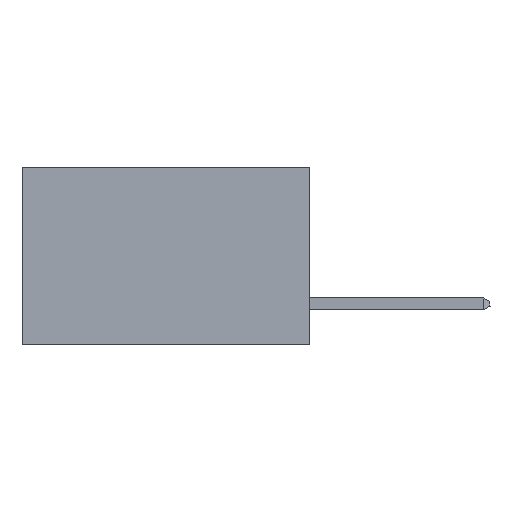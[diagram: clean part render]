
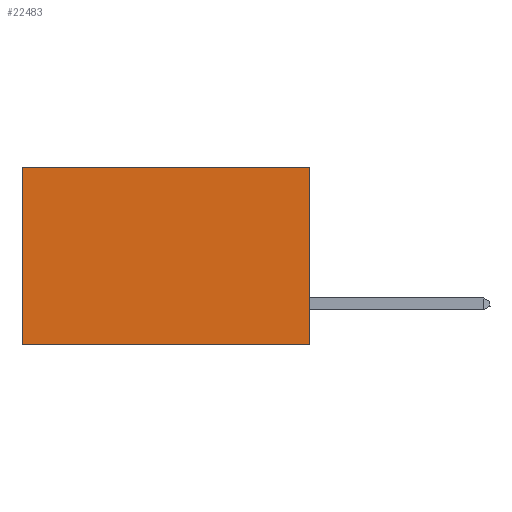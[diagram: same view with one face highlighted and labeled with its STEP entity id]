
A CAD part, left-side view. The second image highlights one B-rep face of the part: STEP entity #22483.
In plain terms, the highlighted planar face has unit normal (-1, 0, 0).
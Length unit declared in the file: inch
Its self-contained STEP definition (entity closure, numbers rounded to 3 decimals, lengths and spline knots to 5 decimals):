
#143 = EDGE_CURVE ( 'NONE', #15144, #19275, #2142, .T. ) ;
#1779 = CARTESIAN_POINT ( 'NONE',  ( 0.2875, 0., 0. ) ) ;
#2142 = LINE ( 'NONE', #35405, #35036 ) ;
#3625 = CARTESIAN_POINT ( 'NONE',  ( 0.2875, 0., 0. ) ) ;
#3890 = CARTESIAN_POINT ( 'NONE',  ( 0.2875, 0.6, 0. ) ) ;
#4076 = VECTOR ( 'NONE', #26128, 39.37008 ) ;
#5432 = ORIENTED_EDGE ( 'NONE', *, *, #30494, .T. ) ;
#9721 = LINE ( 'NONE', #30289, #23962 ) ;
#9836 = ORIENTED_EDGE ( 'NONE', *, *, #143, .F. ) ;
#10707 = DIRECTION ( 'NONE',  ( 0., 0., -1. ) ) ;
#11619 = LINE ( 'NONE', #17474, #4076 ) ;
#12106 = EDGE_CURVE ( 'NONE', #19275, #16424, #9721, .T. ) ;
#12227 = DIRECTION ( 'NONE',  ( 1., 0., 0. ) ) ;
#12586 = EDGE_CURVE ( 'NONE', #32220, #16424, #28326, .T. ) ;
#14504 = VECTOR ( 'NONE', #29594, 39.37008 ) ;
#15144 = VERTEX_POINT ( 'NONE', #1779 ) ;
#16301 = ORIENTED_EDGE ( 'NONE', *, *, #12106, .F. ) ;
#16424 = VERTEX_POINT ( 'NONE', #21352 ) ;
#17474 = CARTESIAN_POINT ( 'NONE',  ( 0.2875, 0., 0. ) ) ;
#17667 = DIRECTION ( 'NONE',  ( 0., 0., -1. ) ) ;
#18583 = CARTESIAN_POINT ( 'NONE',  ( 0.2875, 0.6, 0. ) ) ;
#19146 = DIRECTION ( 'NONE',  ( 0., 1., 0. ) ) ;
#19275 = VERTEX_POINT ( 'NONE', #28253 ) ;
#21352 = CARTESIAN_POINT ( 'NONE',  ( 0.2875, 0.6, -0.37 ) ) ;
#22483 = ADVANCED_FACE ( 'NONE', ( #34348 ), #29214, .F. ) ;
#23962 = VECTOR ( 'NONE', #19146, 39.37008 ) ;
#26128 = DIRECTION ( 'NONE',  ( 0., 1., 0. ) ) ;
#28253 = CARTESIAN_POINT ( 'NONE',  ( 0.2875, 0., -0.37 ) ) ;
#28326 = LINE ( 'NONE', #3890, #14504 ) ;
#29214 = PLANE ( 'NONE',  #31209 ) ;
#29594 = DIRECTION ( 'NONE',  ( 0., 0., -1. ) ) ;
#30289 = CARTESIAN_POINT ( 'NONE',  ( 0.2875, 0., -0.37 ) ) ;
#30494 = EDGE_CURVE ( 'NONE', #15144, #32220, #11619, .T. ) ;
#31209 = AXIS2_PLACEMENT_3D ( 'NONE', #3625, #12227, #17667 ) ;
#32203 = ORIENTED_EDGE ( 'NONE', *, *, #12586, .T. ) ;
#32220 = VERTEX_POINT ( 'NONE', #18583 ) ;
#33221 = EDGE_LOOP ( 'NONE', ( #32203, #16301, #9836, #5432 ) ) ;
#34348 = FACE_OUTER_BOUND ( 'NONE', #33221, .T. ) ;
#35036 = VECTOR ( 'NONE', #10707, 39.37008 ) ;
#35405 = CARTESIAN_POINT ( 'NONE',  ( 0.2875, 0., 0. ) ) ;
